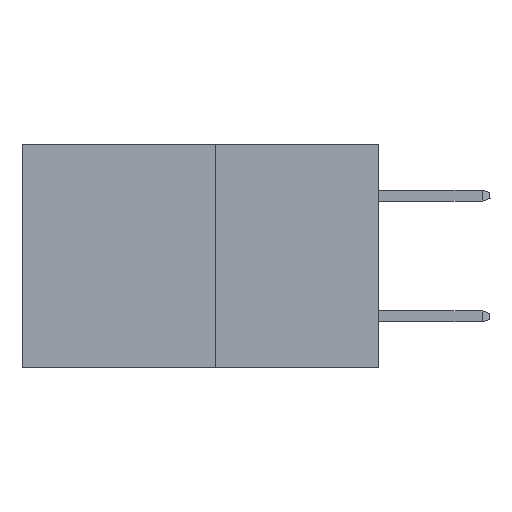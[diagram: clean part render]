
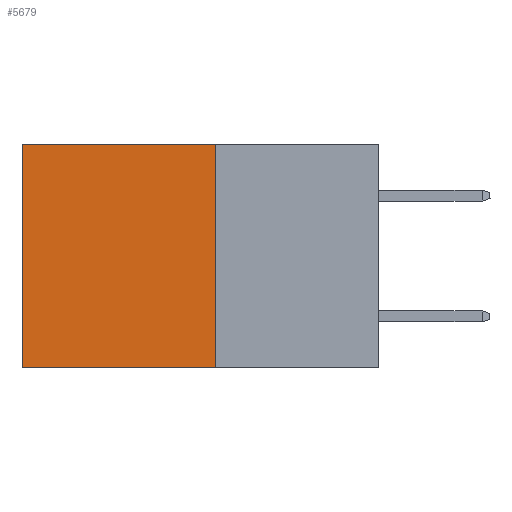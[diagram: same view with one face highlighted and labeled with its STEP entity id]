
A CAD part, left-side view. The second image highlights one B-rep face of the part: STEP entity #5679.
In plain terms, the highlighted planar face has unit normal (-1, 0, 0).
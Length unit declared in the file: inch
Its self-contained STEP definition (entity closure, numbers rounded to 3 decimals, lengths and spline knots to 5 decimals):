
#516 = DIRECTION ( 'NONE',  ( 0., 0., -1. ) ) ;
#1797 = VERTEX_POINT ( 'NONE', #20668 ) ;
#1820 = CARTESIAN_POINT ( 'NONE',  ( 0.277, 0.59, -0.37 ) ) ;
#2292 = PLANE ( 'NONE',  #5928 ) ;
#3630 = EDGE_LOOP ( 'NONE', ( #12028, #15864, #6191, #4626 ) ) ;
#4626 = ORIENTED_EDGE ( 'NONE', *, *, #19172, .T. ) ;
#5193 = VERTEX_POINT ( 'NONE', #14657 ) ;
#5679 = ADVANCED_FACE ( 'NONE', ( #17025 ), #2292, .F. ) ;
#5928 = AXIS2_PLACEMENT_3D ( 'NONE', #8746, #16297, #14617 ) ;
#6191 = ORIENTED_EDGE ( 'NONE', *, *, #9301, .F. ) ;
#6392 = VERTEX_POINT ( 'NONE', #14419 ) ;
#8746 = CARTESIAN_POINT ( 'NONE',  ( 0.277, 0.27, -0.37 ) ) ;
#8811 = LINE ( 'NONE', #1820, #23791 ) ;
#9301 = EDGE_CURVE ( 'NONE', #6392, #1797, #23516, .T. ) ;
#9633 = CARTESIAN_POINT ( 'NONE',  ( 0.277, 0.27, -0.37 ) ) ;
#10029 = CARTESIAN_POINT ( 'NONE',  ( 0.277, 0.27, 0. ) ) ;
#11686 = CARTESIAN_POINT ( 'NONE',  ( 0.277, 0.59, -0.37 ) ) ;
#12028 = ORIENTED_EDGE ( 'NONE', *, *, #13552, .T. ) ;
#13552 = EDGE_CURVE ( 'NONE', #5193, #17571, #8811, .T. ) ;
#13806 = VECTOR ( 'NONE', #516, 39.37008 ) ;
#14419 = CARTESIAN_POINT ( 'NONE',  ( 0.277, 0.27, 0. ) ) ;
#14450 = CARTESIAN_POINT ( 'NONE',  ( 0.277, 0.27, -0.37 ) ) ;
#14617 = DIRECTION ( 'NONE',  ( 0., 0., -1. ) ) ;
#14657 = CARTESIAN_POINT ( 'NONE',  ( 0.277, 0.59, 0. ) ) ;
#15760 = DIRECTION ( 'NONE',  ( 0., 0., -1. ) ) ;
#15864 = ORIENTED_EDGE ( 'NONE', *, *, #20443, .F. ) ;
#16207 = VECTOR ( 'NONE', #19875, 39.37008 ) ;
#16297 = DIRECTION ( 'NONE',  ( 1., 0., 0. ) ) ;
#17025 = FACE_OUTER_BOUND ( 'NONE', #3630, .T. ) ;
#17571 = VERTEX_POINT ( 'NONE', #11686 ) ;
#19172 = EDGE_CURVE ( 'NONE', #6392, #5193, #21373, .T. ) ;
#19875 = DIRECTION ( 'NONE',  ( 0., 1., 0. ) ) ;
#20443 = EDGE_CURVE ( 'NONE', #1797, #17571, #22500, .T. ) ;
#20668 = CARTESIAN_POINT ( 'NONE',  ( 0.277, 0.27, -0.37 ) ) ;
#21373 = LINE ( 'NONE', #10029, #16207 ) ;
#22500 = LINE ( 'NONE', #9633, #23095 ) ;
#23095 = VECTOR ( 'NONE', #23289, 39.37008 ) ;
#23289 = DIRECTION ( 'NONE',  ( 0., 1., 0. ) ) ;
#23516 = LINE ( 'NONE', #14450, #13806 ) ;
#23791 = VECTOR ( 'NONE', #15760, 39.37008 ) ;
